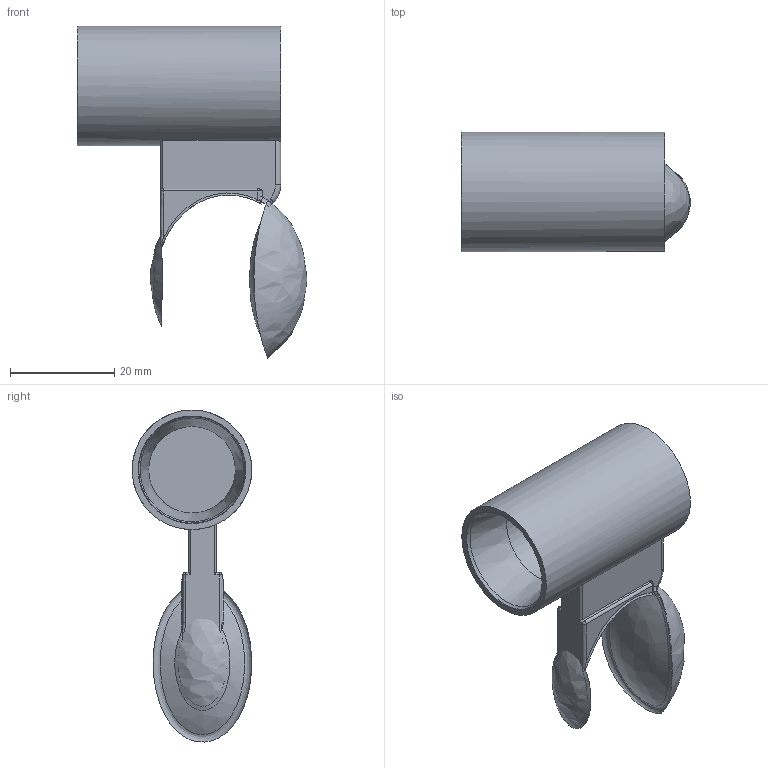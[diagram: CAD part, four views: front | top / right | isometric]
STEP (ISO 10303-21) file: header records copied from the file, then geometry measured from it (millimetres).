
FILE_DESCRIPTION (( 'STEP AP203' ), '1' );
FILE_NAME ('WTF-9MV_charging_handle.STEP', '2020-06-09T21:25:57', ( '' ), ( '' ), 'SwSTEP 2.0', 'SolidWorks 2016', '' );
FILE_SCHEMA (( 'CONFIG_CONTROL_DESIGN' ));
Length unit declared in the file: millimetre
Products named in the file (1): WTF-9MV_charging_handle
Bounding box: 44 x 22.9 x 63.57 mm (x, y, z)
Volume: 9100.4 mm3; surface area: 7194.2 mm2
Topology: 1 solids, 1 shells, 62 faces, 162 edges, 97 vertices
Faces by surface type: bspline 30, cylinder 14, plane 13, sphere 4, cone 1
Full cylindrical faces by diameter (mm): 16.6 x1, 22.9 x1
Entity records: 4948 total; most frequent: CARTESIAN_POINT 3759, ORIENTED_EDGE 286, EDGE_CURVE 143, DIRECTION 120, B_SPLINE_CURVE_WITH_KNOTS 99, VERTEX_POINT 89, EDGE_LOOP 68, FACE_OUTER_BOUND 66
